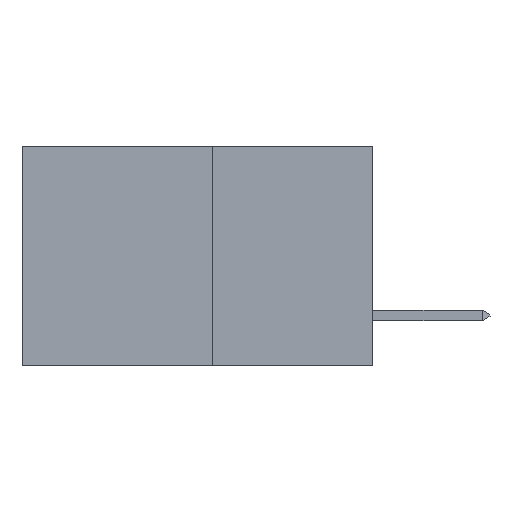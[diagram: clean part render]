
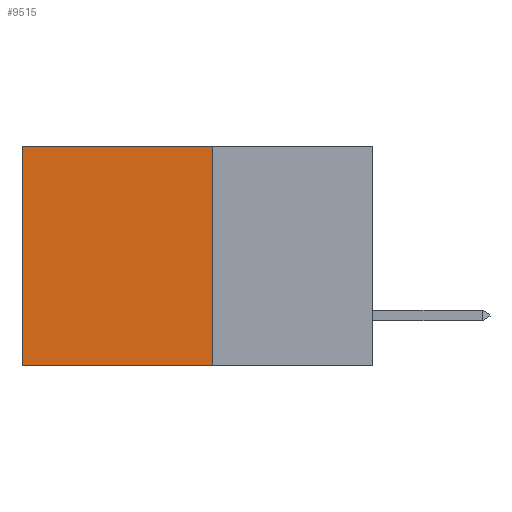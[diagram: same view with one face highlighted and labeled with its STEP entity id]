
A CAD part, left-side view. The second image highlights one B-rep face of the part: STEP entity #9515.
In plain terms, the highlighted planar face has unit normal (-1, 0, 0).
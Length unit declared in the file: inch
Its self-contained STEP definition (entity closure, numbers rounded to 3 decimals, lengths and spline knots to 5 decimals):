
#74 = CARTESIAN_POINT ( 'NONE',  ( 0.277, 0.27, -0.37 ) ) ;
#246 = CARTESIAN_POINT ( 'NONE',  ( 0.277, 0.27, -0.37 ) ) ;
#557 = VERTEX_POINT ( 'NONE', #74 ) ;
#594 = FACE_OUTER_BOUND ( 'NONE', #8591, .T. ) ;
#926 = LINE ( 'NONE', #5254, #9110 ) ;
#1643 = DIRECTION ( 'NONE',  ( 0., 0., -1. ) ) ;
#1741 = CARTESIAN_POINT ( 'NONE',  ( 0.277, 0.27, 0. ) ) ;
#1788 = VERTEX_POINT ( 'NONE', #8066 ) ;
#2631 = DIRECTION ( 'NONE',  ( 0., 0., -1. ) ) ;
#2881 = VERTEX_POINT ( 'NONE', #7771 ) ;
#3269 = VERTEX_POINT ( 'NONE', #7512 ) ;
#4820 = PLANE ( 'NONE',  #6925 ) ;
#4971 = EDGE_CURVE ( 'NONE', #557, #1788, #9373, .T. ) ;
#5141 = VECTOR ( 'NONE', #10258, 39.37008 ) ;
#5206 = EDGE_CURVE ( 'NONE', #2881, #557, #9242, .T. ) ;
#5254 = CARTESIAN_POINT ( 'NONE',  ( 0.277, 0.59, -0.37 ) ) ;
#5321 = LINE ( 'NONE', #1741, #7220 ) ;
#5406 = EDGE_CURVE ( 'NONE', #3269, #1788, #926, .T. ) ;
#5507 = CARTESIAN_POINT ( 'NONE',  ( 0.277, 0.27, -0.37 ) ) ;
#5686 = DIRECTION ( 'NONE',  ( 0., 1., 0. ) ) ;
#6427 = DIRECTION ( 'NONE',  ( 1., 0., 0. ) ) ;
#6925 = AXIS2_PLACEMENT_3D ( 'NONE', #7190, #6427, #1643 ) ;
#7190 = CARTESIAN_POINT ( 'NONE',  ( 0.277, 0.27, -0.37 ) ) ;
#7220 = VECTOR ( 'NONE', #5686, 39.37008 ) ;
#7226 = ORIENTED_EDGE ( 'NONE', *, *, #4971, .F. ) ;
#7388 = VECTOR ( 'NONE', #2631, 39.37008 ) ;
#7406 = ORIENTED_EDGE ( 'NONE', *, *, #7775, .T. ) ;
#7512 = CARTESIAN_POINT ( 'NONE',  ( 0.277, 0.59, 0. ) ) ;
#7771 = CARTESIAN_POINT ( 'NONE',  ( 0.277, 0.27, 0. ) ) ;
#7775 = EDGE_CURVE ( 'NONE', #2881, #3269, #5321, .T. ) ;
#7930 = ORIENTED_EDGE ( 'NONE', *, *, #5406, .T. ) ;
#8066 = CARTESIAN_POINT ( 'NONE',  ( 0.277, 0.59, -0.37 ) ) ;
#8591 = EDGE_LOOP ( 'NONE', ( #7930, #7226, #9873, #7406 ) ) ;
#9110 = VECTOR ( 'NONE', #10022, 39.37008 ) ;
#9242 = LINE ( 'NONE', #246, #7388 ) ;
#9373 = LINE ( 'NONE', #5507, #5141 ) ;
#9515 = ADVANCED_FACE ( 'NONE', ( #594 ), #4820, .F. ) ;
#9873 = ORIENTED_EDGE ( 'NONE', *, *, #5206, .F. ) ;
#10022 = DIRECTION ( 'NONE',  ( 0., 0., -1. ) ) ;
#10258 = DIRECTION ( 'NONE',  ( 0., 1., 0. ) ) ;
